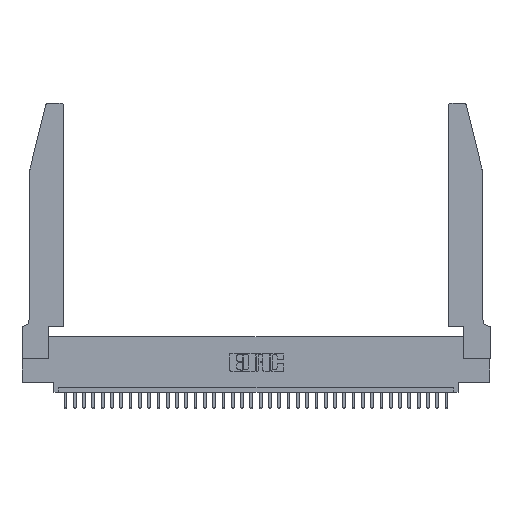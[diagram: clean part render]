
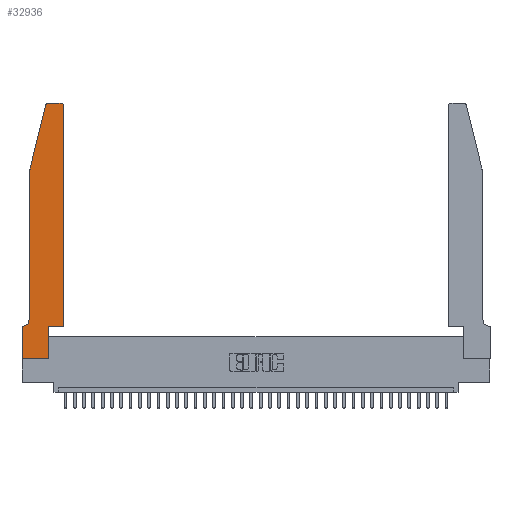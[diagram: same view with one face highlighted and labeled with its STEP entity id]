
A CAD part, top view. The second image highlights one B-rep face of the part: STEP entity #32936.
In plain terms, the highlighted planar face has unit normal (0, 0, 1).
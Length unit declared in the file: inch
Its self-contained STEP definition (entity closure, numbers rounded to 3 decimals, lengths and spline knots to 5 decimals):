
#598 = DIRECTION ( 'NONE',  ( 0., 0., 1. ) ) ;
#1080 = EDGE_CURVE ( 'NONE', #6632, #25015, #26541, .T. ) ;
#1423 = CARTESIAN_POINT ( 'NONE',  ( 0.2865, 0., 0.37 ) ) ;
#1505 = ORIENTED_EDGE ( 'NONE', *, *, #27423, .T. ) ;
#1864 = ORIENTED_EDGE ( 'NONE', *, *, #22807, .T. ) ;
#2015 = CARTESIAN_POINT ( 'NONE',  ( 0.4505, 2.72, 0.37 ) ) ;
#2504 = EDGE_CURVE ( 'NONE', #30664, #27352, #7865, .T. ) ;
#2778 = CARTESIAN_POINT ( 'NONE',  ( 0.0055, 0.42, 0.37 ) ) ;
#2844 = ORIENTED_EDGE ( 'NONE', *, *, #13658, .T. ) ;
#3401 = EDGE_CURVE ( 'NONE', #15369, #9658, #14335, .T. ) ;
#3469 = ORIENTED_EDGE ( 'NONE', *, *, #1080, .T. ) ;
#3713 = EDGE_LOOP ( 'NONE', ( #2844, #31299, #3469, #1505, #12889, #24555, #21986, #33766, #13753, #23535, #1864, #5678 ) ) ;
#4185 = EDGE_CURVE ( 'NONE', #8452, #30664, #23182, .T. ) ;
#4574 = CARTESIAN_POINT ( 'NONE',  ( 0.0755, 0.42, 0.37 ) ) ;
#5000 = VECTOR ( 'NONE', #30819, 39.37008 ) ;
#5678 = ORIENTED_EDGE ( 'NONE', *, *, #17660, .T. ) ;
#6632 = VERTEX_POINT ( 'NONE', #10362 ) ;
#7736 = CIRCLE ( 'NONE', #23447, 0.07 ) ;
#7743 = CARTESIAN_POINT ( 'NONE',  ( 0.2865, 0.35, 0.37 ) ) ;
#7865 = LINE ( 'NONE', #32266, #30441 ) ;
#8452 = VERTEX_POINT ( 'NONE', #15368 ) ;
#8949 = AXIS2_PLACEMENT_3D ( 'NONE', #28958, #15145, #9651 ) ;
#9227 = AXIS2_PLACEMENT_3D ( 'NONE', #23166, #598, #28917 ) ;
#9651 = DIRECTION ( 'NONE',  ( 1., 0., 0. ) ) ;
#9658 = VERTEX_POINT ( 'NONE', #32328 ) ;
#9908 = VECTOR ( 'NONE', #10537, 39.37008 ) ;
#9972 = CARTESIAN_POINT ( 'NONE',  ( 0.4205, 2.72, 0.37 ) ) ;
#10078 = AXIS2_PLACEMENT_3D ( 'NONE', #9972, #18455, #27155 ) ;
#10362 = CARTESIAN_POINT ( 'NONE',  ( 0.25487, 2.72718, 0.37 ) ) ;
#10489 = LINE ( 'NONE', #27792, #30006 ) ;
#10537 = DIRECTION ( 'NONE',  ( 0., -1., 0. ) ) ;
#10813 = CARTESIAN_POINT ( 'NONE',  ( 0.284, 2.75, 0.37 ) ) ;
#11135 = LINE ( 'NONE', #36610, #5000 ) ;
#11331 = CARTESIAN_POINT ( 'NONE',  ( 0.4505, 0.35, 0.37 ) ) ;
#11644 = EDGE_CURVE ( 'NONE', #26721, #15369, #7736, .T. ) ;
#12889 = ORIENTED_EDGE ( 'NONE', *, *, #11644, .T. ) ;
#13263 = CARTESIAN_POINT ( 'NONE',  ( 0.0755, 2., 0.37 ) ) ;
#13658 = EDGE_CURVE ( 'NONE', #32027, #24392, #19912, .T. ) ;
#13753 = ORIENTED_EDGE ( 'NONE', *, *, #2504, .T. ) ;
#13868 = DIRECTION ( 'NONE',  ( 1., 0., 0. ) ) ;
#14335 = LINE ( 'NONE', #29604, #33479 ) ;
#15145 = DIRECTION ( 'NONE',  ( 0., 0., 1. ) ) ;
#15368 = CARTESIAN_POINT ( 'NONE',  ( 0., 0., 0.37 ) ) ;
#15369 = VERTEX_POINT ( 'NONE', #31614 ) ;
#15470 = EDGE_CURVE ( 'NONE', #9658, #8452, #18691, .T. ) ;
#16324 = DIRECTION ( 'NONE',  ( -1., 0., 0. ) ) ;
#16431 = DIRECTION ( 'NONE',  ( 1., 0., 0. ) ) ;
#16831 = DIRECTION ( 'NONE',  ( 0., -1., 0. ) ) ;
#17660 = EDGE_CURVE ( 'NONE', #19079, #32027, #18091, .T. ) ;
#18091 = CIRCLE ( 'NONE', #10078, 0.03 ) ;
#18395 = DIRECTION ( 'NONE',  ( -1., 0., 0. ) ) ;
#18455 = DIRECTION ( 'NONE',  ( 0., 0., 1. ) ) ;
#18691 = LINE ( 'NONE', #32716, #9908 ) ;
#19079 = VERTEX_POINT ( 'NONE', #2015 ) ;
#19520 = CARTESIAN_POINT ( 'NONE',  ( 0.4205, 2.75, 0.37 ) ) ;
#19912 = LINE ( 'NONE', #27651, #33718 ) ;
#20445 = EDGE_CURVE ( 'NONE', #24392, #6632, #24973, .T. ) ;
#21202 = DIRECTION ( 'NONE',  ( -0.239, -0.971, 0. ) ) ;
#21616 = DIRECTION ( 'NONE',  ( 0., 1., 0. ) ) ;
#21986 = ORIENTED_EDGE ( 'NONE', *, *, #15470, .T. ) ;
#22620 = CARTESIAN_POINT ( 'NONE',  ( 0.0755, 2., 0.37 ) ) ;
#22640 = DIRECTION ( 'NONE',  ( 0., 0., -1. ) ) ;
#22807 = EDGE_CURVE ( 'NONE', #25772, #19079, #11135, .T. ) ;
#23045 = PLANE ( 'NONE',  #9227 ) ;
#23166 = CARTESIAN_POINT ( 'NONE',  ( 0., 0.35, 0.37 ) ) ;
#23182 = LINE ( 'NONE', #30183, #29884 ) ;
#23447 = AXIS2_PLACEMENT_3D ( 'NONE', #2778, #22640, #31216 ) ;
#23535 = ORIENTED_EDGE ( 'NONE', *, *, #24345, .T. ) ;
#24251 = FACE_OUTER_BOUND ( 'NONE', #3713, .T. ) ;
#24345 = EDGE_CURVE ( 'NONE', #27352, #25772, #29218, .T. ) ;
#24392 = VERTEX_POINT ( 'NONE', #10813 ) ;
#24555 = ORIENTED_EDGE ( 'NONE', *, *, #3401, .T. ) ;
#24973 = CIRCLE ( 'NONE', #8949, 0.03 ) ;
#25015 = VERTEX_POINT ( 'NONE', #22620 ) ;
#25772 = VERTEX_POINT ( 'NONE', #11331 ) ;
#26541 = LINE ( 'NONE', #13263, #34110 ) ;
#26721 = VERTEX_POINT ( 'NONE', #4574 ) ;
#27155 = DIRECTION ( 'NONE',  ( 1., 0., 0. ) ) ;
#27352 = VERTEX_POINT ( 'NONE', #7743 ) ;
#27423 = EDGE_CURVE ( 'NONE', #25015, #26721, #10489, .T. ) ;
#27651 = CARTESIAN_POINT ( 'NONE',  ( 0.2605, 2.75, 0.37 ) ) ;
#27792 = CARTESIAN_POINT ( 'NONE',  ( 0.0755, 2., 0.37 ) ) ;
#28917 = DIRECTION ( 'NONE',  ( 1., 0., 0. ) ) ;
#28958 = CARTESIAN_POINT ( 'NONE',  ( 0.284, 2.72, 0.37 ) ) ;
#29218 = LINE ( 'NONE', #33513, #36276 ) ;
#29604 = CARTESIAN_POINT ( 'NONE',  ( 0.0755, 0.35, 0.37 ) ) ;
#29884 = VECTOR ( 'NONE', #16431, 39.37008 ) ;
#30006 = VECTOR ( 'NONE', #16831, 39.37008 ) ;
#30183 = CARTESIAN_POINT ( 'NONE',  ( 0., 0., 0.37 ) ) ;
#30441 = VECTOR ( 'NONE', #21616, 39.37008 ) ;
#30664 = VERTEX_POINT ( 'NONE', #1423 ) ;
#30819 = DIRECTION ( 'NONE',  ( 0., 1., 0. ) ) ;
#31216 = DIRECTION ( 'NONE',  ( -1., 0., 0. ) ) ;
#31299 = ORIENTED_EDGE ( 'NONE', *, *, #20445, .T. ) ;
#31614 = CARTESIAN_POINT ( 'NONE',  ( 0.0055, 0.35, 0.37 ) ) ;
#32027 = VERTEX_POINT ( 'NONE', #19520 ) ;
#32266 = CARTESIAN_POINT ( 'NONE',  ( 0.2865, 0.35, 0.37 ) ) ;
#32328 = CARTESIAN_POINT ( 'NONE',  ( 0., 0.35, 0.37 ) ) ;
#32716 = CARTESIAN_POINT ( 'NONE',  ( 0., 0., 0.37 ) ) ;
#32936 = ADVANCED_FACE ( 'NONE', ( #24251 ), #23045, .T. ) ;
#33479 = VECTOR ( 'NONE', #18395, 39.37008 ) ;
#33513 = CARTESIAN_POINT ( 'NONE',  ( 0.4505, 0.35, 0.37 ) ) ;
#33718 = VECTOR ( 'NONE', #16324, 39.37008 ) ;
#33766 = ORIENTED_EDGE ( 'NONE', *, *, #4185, .T. ) ;
#34110 = VECTOR ( 'NONE', #21202, 39.37008 ) ;
#36276 = VECTOR ( 'NONE', #13868, 39.37008 ) ;
#36610 = CARTESIAN_POINT ( 'NONE',  ( 0.4505, 0.35, 0.37 ) ) ;
